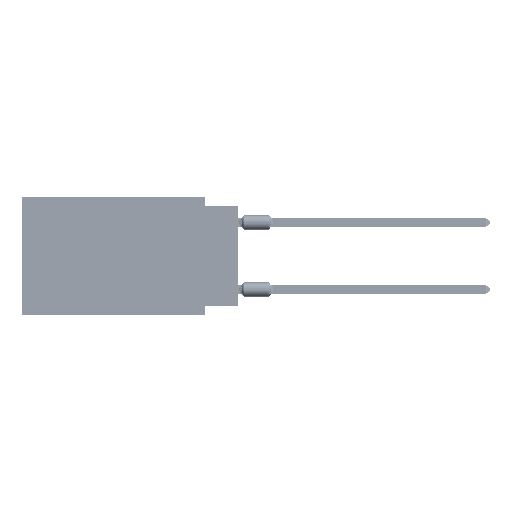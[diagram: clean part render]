
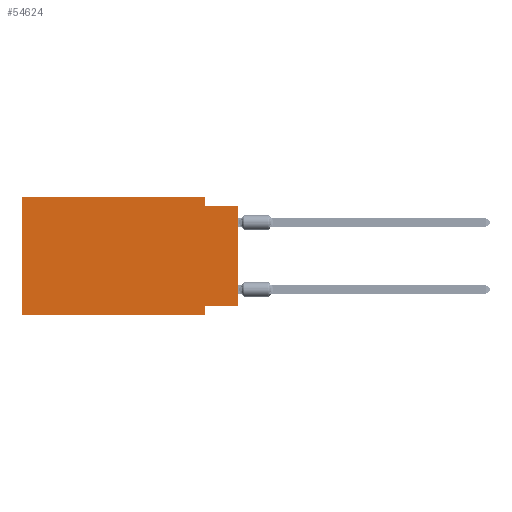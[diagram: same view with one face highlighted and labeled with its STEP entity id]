
A CAD part, left-side view. The second image highlights one B-rep face of the part: STEP entity #54624.
In plain terms, the highlighted planar face has unit normal (-1, 0, 0).
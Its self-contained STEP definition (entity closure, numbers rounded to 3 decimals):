
#6744 = VECTOR ( 'NONE', #97599, 1000. ) ;
#7240 = CARTESIAN_POINT ( 'NONE',  ( 0., 0., -8.255 ) ) ;
#8295 = CARTESIAN_POINT ( 'NONE',  ( 0., 2.54, -8.89 ) ) ;
#12984 = VERTEX_POINT ( 'NONE', #74406 ) ;
#16682 = CARTESIAN_POINT ( 'NONE',  ( 0., 2.54, 0. ) ) ;
#16945 = ORIENTED_EDGE ( 'NONE', *, *, #75191, .F. ) ;
#18449 = ORIENTED_EDGE ( 'NONE', *, *, #79845, .F. ) ;
#20283 = VECTOR ( 'NONE', #84121, 1000. ) ;
#21274 = CARTESIAN_POINT ( 'NONE',  ( 0., 0., -0.635 ) ) ;
#23251 = EDGE_CURVE ( 'NONE', #12984, #51434, #89680, .T. ) ;
#23376 = ORIENTED_EDGE ( 'NONE', *, *, #50975, .F. ) ;
#23757 = EDGE_CURVE ( 'NONE', #73651, #104045, #34387, .T. ) ;
#24295 = ORIENTED_EDGE ( 'NONE', *, *, #104103, .F. ) ;
#25320 = ORIENTED_EDGE ( 'NONE', *, *, #23251, .F. ) ;
#25371 = CARTESIAN_POINT ( 'NONE',  ( 0., 16.383, 0. ) ) ;
#27676 = LINE ( 'NONE', #59888, #39352 ) ;
#29718 = EDGE_CURVE ( 'NONE', #81322, #85971, #76966, .T. ) ;
#32624 = LINE ( 'NONE', #91009, #82716 ) ;
#32907 = CARTESIAN_POINT ( 'NONE',  ( 0., 16.383, 0. ) ) ;
#34387 = LINE ( 'NONE', #68763, #47141 ) ;
#34413 = CARTESIAN_POINT ( 'NONE',  ( 0., 16.383, -8.89 ) ) ;
#37418 = VECTOR ( 'NONE', #95515, 1000. ) ;
#37688 = CARTESIAN_POINT ( 'NONE',  ( 0., 2.54, -0.635 ) ) ;
#39352 = VECTOR ( 'NONE', #94228, 1000. ) ;
#41080 = DIRECTION ( 'NONE',  ( 0., -1., 0. ) ) ;
#42043 = DIRECTION ( 'NONE',  ( 0., -1., 0. ) ) ;
#46756 = CARTESIAN_POINT ( 'NONE',  ( 0., 2.54, -8.89 ) ) ;
#47141 = VECTOR ( 'NONE', #58421, 1000. ) ;
#47419 = CARTESIAN_POINT ( 'NONE',  ( 0., 0., -8.255 ) ) ;
#50975 = EDGE_CURVE ( 'NONE', #51434, #107199, #32624, .T. ) ;
#51434 = VERTEX_POINT ( 'NONE', #16682 ) ;
#54624 = ADVANCED_FACE ( 'NONE', ( #75009 ), #91933, .F. ) ;
#57469 = ORIENTED_EDGE ( 'NONE', *, *, #23757, .T. ) ;
#58421 = DIRECTION ( 'NONE',  ( 0., 0., 1. ) ) ;
#58761 = AXIS2_PLACEMENT_3D ( 'NONE', #25371, #84293, #83747 ) ;
#59888 = CARTESIAN_POINT ( 'NONE',  ( 0., 16.383, 0. ) ) ;
#64709 = EDGE_LOOP ( 'NONE', ( #57469, #16945, #23376, #25320, #76368, #100209, #18449, #24295 ) ) ;
#68134 = VERTEX_POINT ( 'NONE', #105617 ) ;
#68763 = CARTESIAN_POINT ( 'NONE',  ( 0., 0., 0. ) ) ;
#73651 = VERTEX_POINT ( 'NONE', #7240 ) ;
#74406 = CARTESIAN_POINT ( 'NONE',  ( 0., 16.383, 0. ) ) ;
#75009 = FACE_OUTER_BOUND ( 'NONE', #64709, .T. ) ;
#75191 = EDGE_CURVE ( 'NONE', #107199, #104045, #102608, .T. ) ;
#76180 = CARTESIAN_POINT ( 'NONE',  ( 0., 16.383, -8.89 ) ) ;
#76368 = ORIENTED_EDGE ( 'NONE', *, *, #96738, .F. ) ;
#76966 = LINE ( 'NONE', #34413, #77629 ) ;
#77629 = VECTOR ( 'NONE', #42043, 1000. ) ;
#79845 = EDGE_CURVE ( 'NONE', #68134, #85971, #91240, .T. ) ;
#81322 = VERTEX_POINT ( 'NONE', #76180 ) ;
#82716 = VECTOR ( 'NONE', #89944, 1000. ) ;
#83747 = DIRECTION ( 'NONE',  ( 0., 0., -1. ) ) ;
#84121 = DIRECTION ( 'NONE',  ( 0., 0., -1. ) ) ;
#84293 = DIRECTION ( 'NONE',  ( 1., 0., 0. ) ) ;
#85971 = VERTEX_POINT ( 'NONE', #46756 ) ;
#89680 = LINE ( 'NONE', #32907, #92406 ) ;
#89944 = DIRECTION ( 'NONE',  ( 0., 0., -1. ) ) ;
#91009 = CARTESIAN_POINT ( 'NONE',  ( 0., 2.54, 0. ) ) ;
#91240 = LINE ( 'NONE', #8295, #20283 ) ;
#91933 = PLANE ( 'NONE',  #58761 ) ;
#92406 = VECTOR ( 'NONE', #41080, 1000. ) ;
#94228 = DIRECTION ( 'NONE',  ( 0., 0., 1. ) ) ;
#95515 = DIRECTION ( 'NONE',  ( 0., -1., 0. ) ) ;
#96738 = EDGE_CURVE ( 'NONE', #81322, #12984, #27676, .T. ) ;
#97599 = DIRECTION ( 'NONE',  ( 0., 1., 0. ) ) ;
#98141 = LINE ( 'NONE', #47419, #6744 ) ;
#100209 = ORIENTED_EDGE ( 'NONE', *, *, #29718, .T. ) ;
#102608 = LINE ( 'NONE', #103687, #37418 ) ;
#103687 = CARTESIAN_POINT ( 'NONE',  ( 0., 0., -0.635 ) ) ;
#104045 = VERTEX_POINT ( 'NONE', #21274 ) ;
#104103 = EDGE_CURVE ( 'NONE', #73651, #68134, #98141, .T. ) ;
#105617 = CARTESIAN_POINT ( 'NONE',  ( 0., 2.54, -8.255 ) ) ;
#107199 = VERTEX_POINT ( 'NONE', #37688 ) ;
